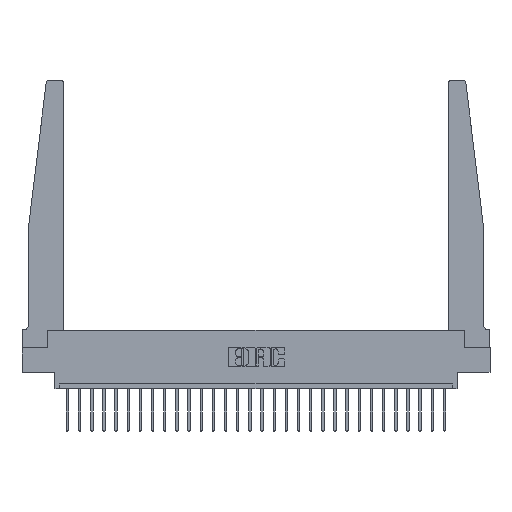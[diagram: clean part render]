
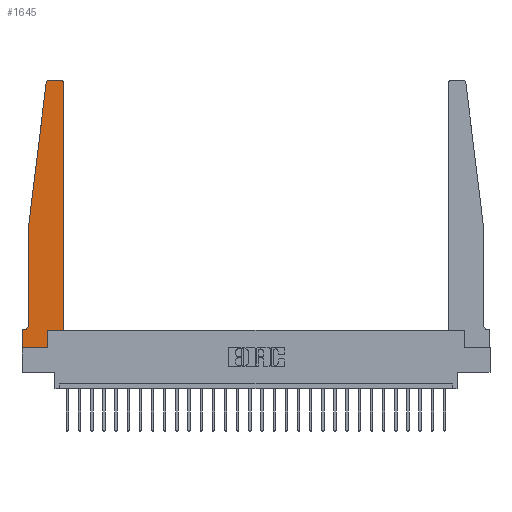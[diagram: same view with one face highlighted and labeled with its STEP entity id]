
A CAD part, top view. The second image highlights one B-rep face of the part: STEP entity #1645.
In plain terms, the highlighted planar face has unit normal (0, 0, 1).
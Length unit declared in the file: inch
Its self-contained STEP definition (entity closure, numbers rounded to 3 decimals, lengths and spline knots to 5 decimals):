
#23 = DIRECTION ( 'NONE',  ( 1., 0., 0. ) ) ;
#147 = CARTESIAN_POINT ( 'NONE',  ( 0., 0., 0.37 ) ) ;
#213 = DIRECTION ( 'NONE',  ( 0., 0., 1. ) ) ;
#302 = CARTESIAN_POINT ( 'NONE',  ( 0.2605, 0., 0.37 ) ) ;
#562 = ORIENTED_EDGE ( 'NONE', *, *, #12155, .T. ) ;
#880 = FACE_OUTER_BOUND ( 'NONE', #9477, .T. ) ;
#1174 = AXIS2_PLACEMENT_3D ( 'NONE', #16726, #23192, #10571 ) ;
#1259 = CARTESIAN_POINT ( 'NONE',  ( 0.065, 0.1875, 0.37 ) ) ;
#1581 = CARTESIAN_POINT ( 'NONE',  ( 0.2605, 0.18, 0.37 ) ) ;
#1645 = ADVANCED_FACE ( 'NONE', ( #880 ), #25043, .T. ) ;
#2064 = VERTEX_POINT ( 'NONE', #25389 ) ;
#2533 = VERTEX_POINT ( 'NONE', #13707 ) ;
#2652 = DIRECTION ( 'NONE',  ( 1., 0., 0. ) ) ;
#2928 = VECTOR ( 'NONE', #12683, 39.37008 ) ;
#3044 = VERTEX_POINT ( 'NONE', #26285 ) ;
#3086 = ORIENTED_EDGE ( 'NONE', *, *, #8063, .T. ) ;
#3460 = DIRECTION ( 'NONE',  ( -1., 0., 0. ) ) ;
#3614 = DIRECTION ( 'NONE',  ( 0., 1., 0. ) ) ;
#4380 = LINE ( 'NONE', #20734, #2928 ) ;
#4580 = CARTESIAN_POINT ( 'NONE',  ( 0.395, 2.72, 0.37 ) ) ;
#4593 = VECTOR ( 'NONE', #13665, 39.37008 ) ;
#4745 = ORIENTED_EDGE ( 'NONE', *, *, #10158, .T. ) ;
#5163 = EDGE_CURVE ( 'NONE', #7883, #20893, #18568, .T. ) ;
#5497 = CARTESIAN_POINT ( 'NONE',  ( 0.065, 1.25, 0.37 ) ) ;
#6538 = VERTEX_POINT ( 'NONE', #15279 ) ;
#6561 = ORIENTED_EDGE ( 'NONE', *, *, #12017, .T. ) ;
#6678 = EDGE_CURVE ( 'NONE', #2533, #15357, #22000, .T. ) ;
#6790 = VERTEX_POINT ( 'NONE', #22124 ) ;
#6948 = DIRECTION ( 'NONE',  ( -1., 0., 0. ) ) ;
#6976 = VECTOR ( 'NONE', #3614, 39.37008 ) ;
#7209 = LINE ( 'NONE', #1259, #20068 ) ;
#7515 = ORIENTED_EDGE ( 'NONE', *, *, #16865, .T. ) ;
#7883 = VERTEX_POINT ( 'NONE', #16906 ) ;
#8063 = EDGE_CURVE ( 'NONE', #3044, #6538, #10185, .T. ) ;
#8923 = CIRCLE ( 'NONE', #1174, 0.05 ) ;
#9477 = EDGE_LOOP ( 'NONE', ( #18385, #3086, #17986, #4745, #13045, #17583, #20978, #562, #16978, #7515, #18182, #6561 ) ) ;
#9842 = AXIS2_PLACEMENT_3D ( 'NONE', #14978, #23037, #2652 ) ;
#10158 = EDGE_CURVE ( 'NONE', #6790, #2064, #19185, .T. ) ;
#10185 = CIRCLE ( 'NONE', #12750, 0.03 ) ;
#10290 = DIRECTION ( 'NONE',  ( 1., 0., 0. ) ) ;
#10462 = EDGE_CURVE ( 'NONE', #2064, #17877, #8923, .T. ) ;
#10571 = DIRECTION ( 'NONE',  ( -1., 0., 0. ) ) ;
#10950 = EDGE_CURVE ( 'NONE', #6538, #6790, #4380, .T. ) ;
#11110 = VECTOR ( 'NONE', #25005, 39.37008 ) ;
#11126 = EDGE_CURVE ( 'NONE', #17877, #7883, #7209, .T. ) ;
#11195 = VECTOR ( 'NONE', #18970, 39.37008 ) ;
#11226 = CARTESIAN_POINT ( 'NONE',  ( 0.015, 0.1875, 0.37 ) ) ;
#12017 = EDGE_CURVE ( 'NONE', #15357, #13267, #23538, .T. ) ;
#12155 = EDGE_CURVE ( 'NONE', #20893, #19410, #15914, .T. ) ;
#12595 = VECTOR ( 'NONE', #23, 39.37008 ) ;
#12683 = DIRECTION ( 'NONE',  ( -0.122, -0.992, 0. ) ) ;
#12750 = AXIS2_PLACEMENT_3D ( 'NONE', #26418, #213, #18628 ) ;
#12757 = DIRECTION ( 'NONE',  ( 1., 0., 0. ) ) ;
#13045 = ORIENTED_EDGE ( 'NONE', *, *, #10462, .T. ) ;
#13267 = VERTEX_POINT ( 'NONE', #25097 ) ;
#13665 = DIRECTION ( 'NONE',  ( 0., -1., 0. ) ) ;
#13707 = CARTESIAN_POINT ( 'NONE',  ( 0.425, 0.18, 0.37 ) ) ;
#14056 = VECTOR ( 'NONE', #3460, 39.37008 ) ;
#14264 = LINE ( 'NONE', #16532, #12595 ) ;
#14978 = CARTESIAN_POINT ( 'NONE',  ( 0., 0.1875, 0.37 ) ) ;
#15279 = CARTESIAN_POINT ( 'NONE',  ( 0.24675, 2.72367, 0.37 ) ) ;
#15357 = VERTEX_POINT ( 'NONE', #25271 ) ;
#15539 = CARTESIAN_POINT ( 'NONE',  ( 0.425, 0.18, 0.37 ) ) ;
#15914 = LINE ( 'NONE', #16169, #19246 ) ;
#16169 = CARTESIAN_POINT ( 'NONE',  ( 0., 0., 0.37 ) ) ;
#16234 = AXIS2_PLACEMENT_3D ( 'NONE', #4580, #22951, #12757 ) ;
#16532 = CARTESIAN_POINT ( 'NONE',  ( 0.425, 0.18, 0.37 ) ) ;
#16726 = CARTESIAN_POINT ( 'NONE',  ( 0.015, 0.2375, 0.37 ) ) ;
#16865 = EDGE_CURVE ( 'NONE', #21818, #2533, #14264, .T. ) ;
#16906 = CARTESIAN_POINT ( 'NONE',  ( 0., 0.1875, 0.37 ) ) ;
#16978 = ORIENTED_EDGE ( 'NONE', *, *, #25428, .T. ) ;
#17276 = CARTESIAN_POINT ( 'NONE',  ( 0.25, 2.75, 0.37 ) ) ;
#17539 = LINE ( 'NONE', #17276, #14056 ) ;
#17583 = ORIENTED_EDGE ( 'NONE', *, *, #11126, .T. ) ;
#17877 = VERTEX_POINT ( 'NONE', #11226 ) ;
#17986 = ORIENTED_EDGE ( 'NONE', *, *, #10950, .T. ) ;
#18182 = ORIENTED_EDGE ( 'NONE', *, *, #6678, .T. ) ;
#18385 = ORIENTED_EDGE ( 'NONE', *, *, #24747, .T. ) ;
#18568 = LINE ( 'NONE', #147, #11195 ) ;
#18628 = DIRECTION ( 'NONE',  ( 1., 0., 0. ) ) ;
#18970 = DIRECTION ( 'NONE',  ( 0., -1., 0. ) ) ;
#19185 = LINE ( 'NONE', #5497, #4593 ) ;
#19246 = VECTOR ( 'NONE', #10290, 39.37008 ) ;
#19410 = VERTEX_POINT ( 'NONE', #302 ) ;
#20068 = VECTOR ( 'NONE', #6948, 39.37008 ) ;
#20734 = CARTESIAN_POINT ( 'NONE',  ( 0.065, 1.25, 0.37 ) ) ;
#20846 = LINE ( 'NONE', #22592, #11110 ) ;
#20893 = VERTEX_POINT ( 'NONE', #25687 ) ;
#20978 = ORIENTED_EDGE ( 'NONE', *, *, #5163, .T. ) ;
#21818 = VERTEX_POINT ( 'NONE', #1581 ) ;
#22000 = LINE ( 'NONE', #15539, #6976 ) ;
#22124 = CARTESIAN_POINT ( 'NONE',  ( 0.065, 1.25, 0.37 ) ) ;
#22592 = CARTESIAN_POINT ( 'NONE',  ( 0.2605, 0.18, 0.37 ) ) ;
#22951 = DIRECTION ( 'NONE',  ( 0., 0., 1. ) ) ;
#23037 = DIRECTION ( 'NONE',  ( 0., 0., 1. ) ) ;
#23192 = DIRECTION ( 'NONE',  ( 0., 0., -1. ) ) ;
#23538 = CIRCLE ( 'NONE', #16234, 0.03 ) ;
#24747 = EDGE_CURVE ( 'NONE', #13267, #3044, #17539, .T. ) ;
#25005 = DIRECTION ( 'NONE',  ( 0., 1., 0. ) ) ;
#25043 = PLANE ( 'NONE',  #9842 ) ;
#25097 = CARTESIAN_POINT ( 'NONE',  ( 0.395, 2.75, 0.37 ) ) ;
#25271 = CARTESIAN_POINT ( 'NONE',  ( 0.425, 2.72, 0.37 ) ) ;
#25389 = CARTESIAN_POINT ( 'NONE',  ( 0.065, 0.2375, 0.37 ) ) ;
#25428 = EDGE_CURVE ( 'NONE', #19410, #21818, #20846, .T. ) ;
#25687 = CARTESIAN_POINT ( 'NONE',  ( 0., 0., 0.37 ) ) ;
#26285 = CARTESIAN_POINT ( 'NONE',  ( 0.27653, 2.75, 0.37 ) ) ;
#26418 = CARTESIAN_POINT ( 'NONE',  ( 0.27653, 2.72, 0.37 ) ) ;
